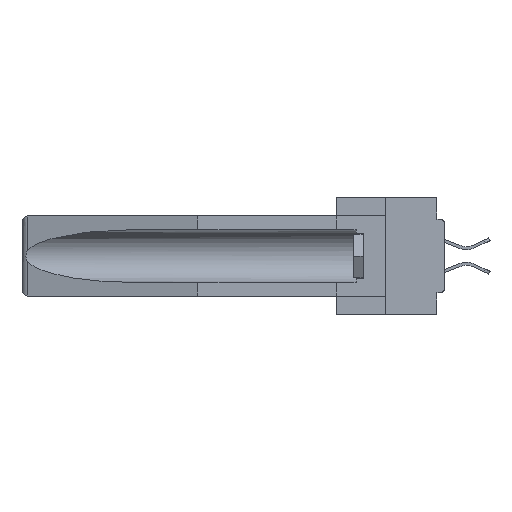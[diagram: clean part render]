
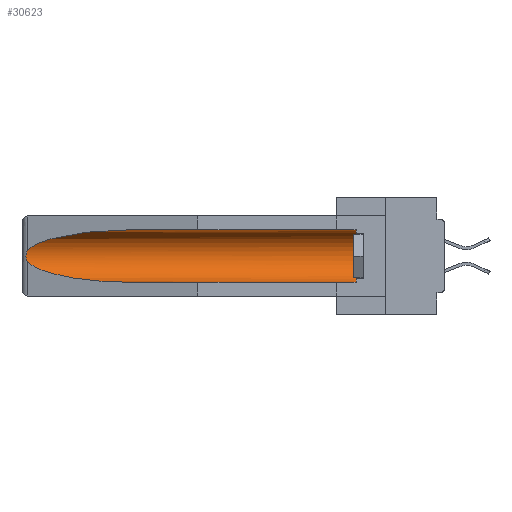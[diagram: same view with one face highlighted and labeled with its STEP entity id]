
A CAD part, left-side view. The second image highlights one B-rep face of the part: STEP entity #30623.
In plain terms, the highlighted cylindrical face has radius 2.857 mm (diameter 5.715 mm), a partial arc.
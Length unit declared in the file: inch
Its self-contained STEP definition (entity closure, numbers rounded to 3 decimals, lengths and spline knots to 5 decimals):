
#940 = LINE ( 'NONE', #23909, #16535 ) ;
#975 = CARTESIAN_POINT ( 'NONE',  ( 0.26655, 1.53094, -0.18657 ) ) ;
#1471 =( BOUNDED_CURVE ( )  B_SPLINE_CURVE ( 3, ( #2476, #8629, #18139, #8766 ),
 .UNSPECIFIED., .F., .F. ) 
 B_SPLINE_CURVE_WITH_KNOTS ( ( 4, 4 ),
 ( 0.1948, 1.5708 ),
 .UNSPECIFIED. ) 
 CURVE ( )  GEOMETRIC_REPRESENTATION_ITEM ( )  RATIONAL_B_SPLINE_CURVE ( ( 1., 0.848, 0.848, 1. ) ) 
 REPRESENTATION_ITEM ( '' )  );
#2175 = CARTESIAN_POINT ( 'NONE',  ( 0.21114, 1.30732, -0.059 ) ) ;
#2476 = CARTESIAN_POINT ( 'NONE',  ( 0.26537, 1.52718, -0.19328 ) ) ;
#2998 = CARTESIAN_POINT ( 'NONE',  ( 0.155, 0.126, -0.284 ) ) ;
#3970 = CARTESIAN_POINT ( 'NONE',  ( 0.26597, 1.52961, -0.15275 ) ) ;
#5629 = ORIENTED_EDGE ( 'NONE', *, *, #37249, .F. ) ;
#5853 = VERTEX_POINT ( 'NONE', #2998 ) ;
#6128 = CARTESIAN_POINT ( 'NONE',  ( 0.155, 1.07973, -0.059 ) ) ;
#6950 = CARTESIAN_POINT ( 'NONE',  ( 0.155, 0.126, -0.1715 ) ) ;
#7118 = CARTESIAN_POINT ( 'NONE',  ( 0.155, -0.30754, -0.284 ) ) ;
#7923 = LINE ( 'NONE', #7118, #23565 ) ;
#8629 = CARTESIAN_POINT ( 'NONE',  ( 0.25451, 1.48313, -0.24835 ) ) ;
#8766 = CARTESIAN_POINT ( 'NONE',  ( 0.155, 1.07973, -0.284 ) ) ;
#10264 = EDGE_CURVE ( 'NONE', #19290, #19287, #15960, .T. ) ;
#11852 = DIRECTION ( 'NONE',  ( 0., 1., 0. ) ) ;
#12125 = CIRCLE ( 'NONE', #13430, 0.1125 ) ;
#12502 = VERTEX_POINT ( 'NONE', #30114 ) ;
#13430 = AXIS2_PLACEMENT_3D ( 'NONE', #6950, #22819, #25926 ) ;
#14273 = CYLINDRICAL_SURFACE ( 'NONE', #22682, 0.1125 ) ;
#14879 = CARTESIAN_POINT ( 'NONE',  ( 0.155, 0.126, -0.059 ) ) ;
#15960 = B_SPLINE_CURVE_WITH_KNOTS ( 'NONE', 3,
 ( #25672, #3970, #38119, #34981, #16767, #29077, #19371, #975, #32221, #32356 ),
 .UNSPECIFIED., .F., .F.,
 ( 4, 2, 2, 2, 4 ),
 ( 0., 0.00029, 0.00058, 0.00087, 0.00117 ),
 .UNSPECIFIED. ) ;
#16263 = DIRECTION ( 'NONE',  ( 0., 1., 0. ) ) ;
#16460 = EDGE_CURVE ( 'NONE', #18101, #32164, #940, .T. ) ;
#16535 = VECTOR ( 'NONE', #11852, 39.37008 ) ;
#16767 = CARTESIAN_POINT ( 'NONE',  ( 0.2675, 1.53308, -0.16763 ) ) ;
#18101 = VERTEX_POINT ( 'NONE', #14879 ) ;
#18139 = CARTESIAN_POINT ( 'NONE',  ( 0.21114, 1.30732, -0.284 ) ) ;
#19287 = VERTEX_POINT ( 'NONE', #38319 ) ;
#19290 = VERTEX_POINT ( 'NONE', #25863 ) ;
#19371 = CARTESIAN_POINT ( 'NONE',  ( 0.2673, 1.53269, -0.17917 ) ) ;
#20446 = CARTESIAN_POINT ( 'NONE',  ( 0.25451, 1.48313, -0.09465 ) ) ;
#21786 = DIRECTION ( 'NONE',  ( 0., 1., 0. ) ) ;
#22516 = ORIENTED_EDGE ( 'NONE', *, *, #10264, .T. ) ;
#22682 = AXIS2_PLACEMENT_3D ( 'NONE', #25332, #21786, #35692 ) ;
#22819 = DIRECTION ( 'NONE',  ( 0., -1., 0. ) ) ;
#23565 = VECTOR ( 'NONE', #16263, 39.37008 ) ;
#23909 = CARTESIAN_POINT ( 'NONE',  ( 0.155, -0.30754, -0.059 ) ) ;
#25332 = CARTESIAN_POINT ( 'NONE',  ( 0.155, -0.30754, -0.1715 ) ) ;
#25672 = CARTESIAN_POINT ( 'NONE',  ( 0.26537, 1.52718, -0.14972 ) ) ;
#25731 =( BOUNDED_CURVE ( )  B_SPLINE_CURVE ( 3, ( #39169, #2175, #20446, #39311 ),
 .UNSPECIFIED., .F., .F. ) 
 B_SPLINE_CURVE_WITH_KNOTS ( ( 4, 4 ),
 ( 4.71239, 6.08839 ),
 .UNSPECIFIED. ) 
 CURVE ( )  GEOMETRIC_REPRESENTATION_ITEM ( )  RATIONAL_B_SPLINE_CURVE ( ( 1., 0.848, 0.848, 1. ) ) 
 REPRESENTATION_ITEM ( '' )  );
#25863 = CARTESIAN_POINT ( 'NONE',  ( 0.26537, 1.52718, -0.14972 ) ) ;
#25926 = DIRECTION ( 'NONE',  ( 0., 0., 1. ) ) ;
#26508 = FACE_OUTER_BOUND ( 'NONE', #27001, .T. ) ;
#27001 = EDGE_LOOP ( 'NONE', ( #32932, #22516, #36145, #5629, #37785, #30191 ) ) ;
#27688 = EDGE_CURVE ( 'NONE', #32164, #19290, #25731, .T. ) ;
#28250 = EDGE_CURVE ( 'NONE', #19287, #12502, #1471, .T. ) ;
#29077 = CARTESIAN_POINT ( 'NONE',  ( 0.2675, 1.53308, -0.17534 ) ) ;
#30114 = CARTESIAN_POINT ( 'NONE',  ( 0.155, 1.07973, -0.284 ) ) ;
#30191 = ORIENTED_EDGE ( 'NONE', *, *, #16460, .T. ) ;
#30623 = ADVANCED_FACE ( 'NONE', ( #26508 ), #14273, .F. ) ;
#32164 = VERTEX_POINT ( 'NONE', #6128 ) ;
#32221 = CARTESIAN_POINT ( 'NONE',  ( 0.26597, 1.5296, -0.19026 ) ) ;
#32356 = CARTESIAN_POINT ( 'NONE',  ( 0.26537, 1.52718, -0.19328 ) ) ;
#32932 = ORIENTED_EDGE ( 'NONE', *, *, #27688, .T. ) ;
#34981 = CARTESIAN_POINT ( 'NONE',  ( 0.2673, 1.5327, -0.16383 ) ) ;
#35692 = DIRECTION ( 'NONE',  ( 0., 0., 1. ) ) ;
#36145 = ORIENTED_EDGE ( 'NONE', *, *, #28250, .T. ) ;
#37249 = EDGE_CURVE ( 'NONE', #5853, #12502, #7923, .T. ) ;
#37785 = ORIENTED_EDGE ( 'NONE', *, *, #39751, .T. ) ;
#38119 = CARTESIAN_POINT ( 'NONE',  ( 0.26654, 1.53092, -0.15636 ) ) ;
#38319 = CARTESIAN_POINT ( 'NONE',  ( 0.26537, 1.52718, -0.19328 ) ) ;
#39169 = CARTESIAN_POINT ( 'NONE',  ( 0.155, 1.07973, -0.059 ) ) ;
#39311 = CARTESIAN_POINT ( 'NONE',  ( 0.26537, 1.52718, -0.14972 ) ) ;
#39751 = EDGE_CURVE ( 'NONE', #5853, #18101, #12125, .T. ) ;
